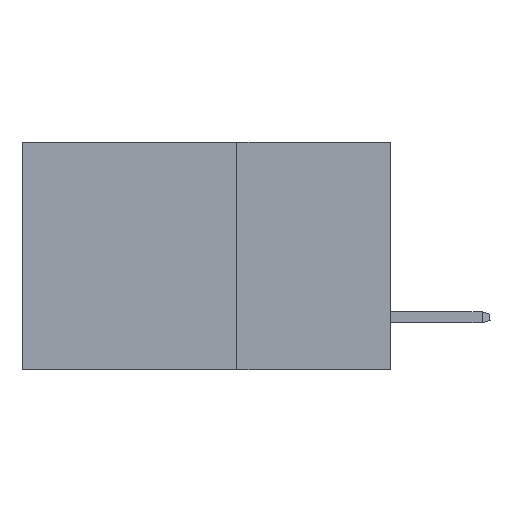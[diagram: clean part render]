
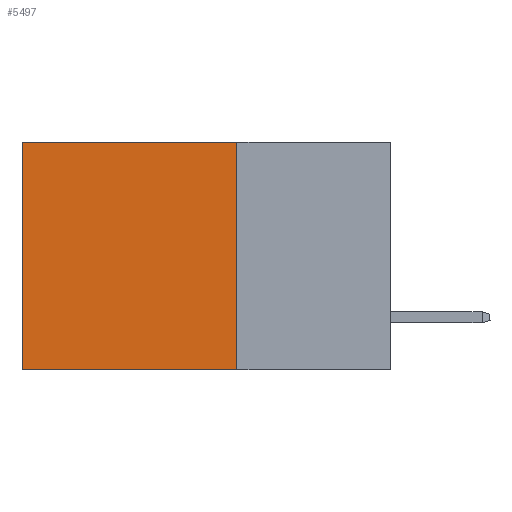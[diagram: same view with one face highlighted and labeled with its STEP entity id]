
A CAD part, left-side view. The second image highlights one B-rep face of the part: STEP entity #5497.
In plain terms, the highlighted planar face has unit normal (-1, 0, 0).
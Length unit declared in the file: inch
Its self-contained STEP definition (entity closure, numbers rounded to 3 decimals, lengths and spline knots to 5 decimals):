
#1055 = VECTOR ( 'NONE', #24900, 39.37008 ) ;
#5497 = ADVANCED_FACE ( 'NONE', ( #19946 ), #7611, .F. ) ;
#6565 = EDGE_CURVE ( 'NONE', #16283, #29024, #14775, .T. ) ;
#7304 = DIRECTION ( 'NONE',  ( 1., 0., 0. ) ) ;
#7611 = PLANE ( 'NONE',  #32080 ) ;
#8221 = DIRECTION ( 'NONE',  ( 0., 0., -1. ) ) ;
#8757 = EDGE_LOOP ( 'NONE', ( #27594, #11748, #26244, #14573 ) ) ;
#10108 = CARTESIAN_POINT ( 'NONE',  ( 0.2875, 0.25, 0. ) ) ;
#10478 = CARTESIAN_POINT ( 'NONE',  ( 0.2875, 0.6, -0.37 ) ) ;
#10508 = EDGE_CURVE ( 'NONE', #19645, #16283, #28531, .T. ) ;
#11736 = DIRECTION ( 'NONE',  ( 0., 1., 0. ) ) ;
#11748 = ORIENTED_EDGE ( 'NONE', *, *, #16877, .F. ) ;
#11831 = CARTESIAN_POINT ( 'NONE',  ( 0.2875, 0.6, 0. ) ) ;
#11887 = CARTESIAN_POINT ( 'NONE',  ( 0.2875, 0.25, -0.37 ) ) ;
#12003 = CARTESIAN_POINT ( 'NONE',  ( 0.2875, 0.6, 0. ) ) ;
#14432 = CARTESIAN_POINT ( 'NONE',  ( 0.2875, 0.25, 0. ) ) ;
#14573 = ORIENTED_EDGE ( 'NONE', *, *, #10508, .T. ) ;
#14775 = LINE ( 'NONE', #11831, #1055 ) ;
#14825 = VECTOR ( 'NONE', #11736, 39.37008 ) ;
#16283 = VERTEX_POINT ( 'NONE', #12003 ) ;
#16877 = EDGE_CURVE ( 'NONE', #22661, #29024, #24711, .T. ) ;
#18787 = CARTESIAN_POINT ( 'NONE',  ( 0.2875, 0.25, 0. ) ) ;
#19645 = VERTEX_POINT ( 'NONE', #31855 ) ;
#19946 = FACE_OUTER_BOUND ( 'NONE', #8757, .T. ) ;
#20571 = LINE ( 'NONE', #18787, #30294 ) ;
#22661 = VERTEX_POINT ( 'NONE', #22831 ) ;
#22831 = CARTESIAN_POINT ( 'NONE',  ( 0.2875, 0.25, -0.37 ) ) ;
#23433 = VECTOR ( 'NONE', #25081, 39.37008 ) ;
#24711 = LINE ( 'NONE', #11887, #23433 ) ;
#24900 = DIRECTION ( 'NONE',  ( 0., 0., -1. ) ) ;
#25081 = DIRECTION ( 'NONE',  ( 0., 1., 0. ) ) ;
#25301 = DIRECTION ( 'NONE',  ( 0., 0., -1. ) ) ;
#26244 = ORIENTED_EDGE ( 'NONE', *, *, #27303, .F. ) ;
#27303 = EDGE_CURVE ( 'NONE', #19645, #22661, #20571, .T. ) ;
#27594 = ORIENTED_EDGE ( 'NONE', *, *, #6565, .T. ) ;
#28531 = LINE ( 'NONE', #14432, #14825 ) ;
#29024 = VERTEX_POINT ( 'NONE', #10478 ) ;
#30294 = VECTOR ( 'NONE', #8221, 39.37008 ) ;
#31855 = CARTESIAN_POINT ( 'NONE',  ( 0.2875, 0.25, 0. ) ) ;
#32080 = AXIS2_PLACEMENT_3D ( 'NONE', #10108, #7304, #25301 ) ;
